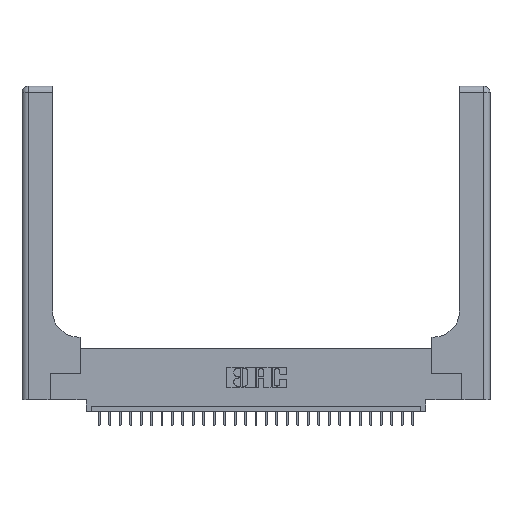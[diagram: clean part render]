
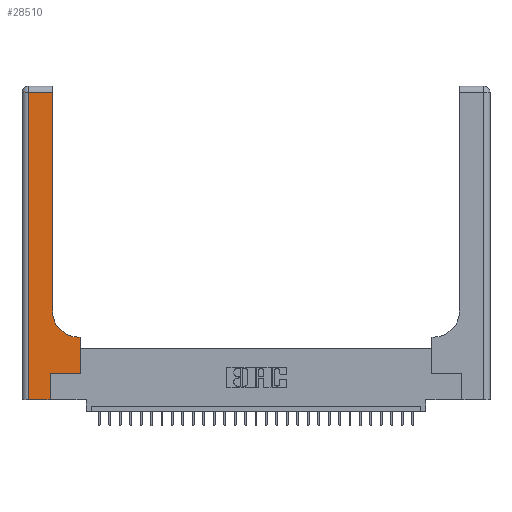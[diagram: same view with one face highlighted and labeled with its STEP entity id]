
A CAD part, top view. The second image highlights one B-rep face of the part: STEP entity #28510.
In plain terms, the highlighted planar face has unit normal (0, 0, 1).
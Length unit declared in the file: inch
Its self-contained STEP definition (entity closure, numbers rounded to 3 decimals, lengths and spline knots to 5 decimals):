
#243 = CARTESIAN_POINT ( 'NONE',  ( 0.269, 0.25, 0.37 ) ) ;
#342 = VERTEX_POINT ( 'NONE', #17810 ) ;
#638 = DIRECTION ( 'NONE',  ( 1., 0., 0. ) ) ;
#1410 = VECTOR ( 'NONE', #7088, 39.37008 ) ;
#2041 = EDGE_CURVE ( 'NONE', #10091, #8003, #2629, .T. ) ;
#2629 = LINE ( 'NONE', #28182, #18764 ) ;
#3661 = CARTESIAN_POINT ( 'NONE',  ( 0.269, 0., 0.37 ) ) ;
#4192 = ORIENTED_EDGE ( 'NONE', *, *, #15977, .T. ) ;
#4595 = EDGE_LOOP ( 'NONE', ( #4192, #26005, #29507, #8816, #28976, #13004, #23327, #13872, #29586 ) ) ;
#4893 = VECTOR ( 'NONE', #10090, 39.37008 ) ;
#5829 = DIRECTION ( 'NONE',  ( 0., -1., 0. ) ) ;
#6194 = CIRCLE ( 'NONE', #23315, 0.25 ) ;
#6256 = EDGE_CURVE ( 'NONE', #19738, #10091, #20917, .T. ) ;
#6762 = DIRECTION ( 'NONE',  ( -1., 0., 0. ) ) ;
#7088 = DIRECTION ( 'NONE',  ( -1., 0., 0. ) ) ;
#7110 = VECTOR ( 'NONE', #6762, 39.37008 ) ;
#7513 = VERTEX_POINT ( 'NONE', #15876 ) ;
#7803 = FACE_OUTER_BOUND ( 'NONE', #4595, .T. ) ;
#8003 = VERTEX_POINT ( 'NONE', #16658 ) ;
#8239 = LINE ( 'NONE', #26913, #28339 ) ;
#8816 = ORIENTED_EDGE ( 'NONE', *, *, #11697, .T. ) ;
#9368 = LINE ( 'NONE', #18712, #1410 ) ;
#9476 = CARTESIAN_POINT ( 'NONE',  ( 0.06, 2.94, 0.37 ) ) ;
#9731 = CARTESIAN_POINT ( 'NONE',  ( 0.269, 0., 0.37 ) ) ;
#10090 = DIRECTION ( 'NONE',  ( 0., 1., 0. ) ) ;
#10091 = VERTEX_POINT ( 'NONE', #243 ) ;
#10159 = CARTESIAN_POINT ( 'NONE',  ( 0.2915, 2.94, 0.37 ) ) ;
#10272 = EDGE_CURVE ( 'NONE', #14454, #7513, #6194, .T. ) ;
#11044 = LINE ( 'NONE', #30011, #7110 ) ;
#11697 = EDGE_CURVE ( 'NONE', #342, #19738, #15534, .T. ) ;
#12096 = VERTEX_POINT ( 'NONE', #9476 ) ;
#12359 = VECTOR ( 'NONE', #14035, 39.37008 ) ;
#13004 = ORIENTED_EDGE ( 'NONE', *, *, #2041, .T. ) ;
#13872 = ORIENTED_EDGE ( 'NONE', *, *, #29369, .T. ) ;
#14035 = DIRECTION ( 'NONE',  ( 0., 1., 0. ) ) ;
#14454 = VERTEX_POINT ( 'NONE', #27743 ) ;
#14844 = DIRECTION ( 'NONE',  ( 0., 0., -1. ) ) ;
#14993 = LINE ( 'NONE', #24343, #4893 ) ;
#15042 = CARTESIAN_POINT ( 'NONE',  ( 0.5415, 0.85, 0.37 ) ) ;
#15534 = LINE ( 'NONE', #25197, #23855 ) ;
#15876 = CARTESIAN_POINT ( 'NONE',  ( 0.2915, 0.85, 0.37 ) ) ;
#15977 = EDGE_CURVE ( 'NONE', #7513, #16797, #8239, .T. ) ;
#16658 = CARTESIAN_POINT ( 'NONE',  ( 0.5585, 0.25, 0.37 ) ) ;
#16797 = VERTEX_POINT ( 'NONE', #10159 ) ;
#17145 = PLANE ( 'NONE',  #23704 ) ;
#17810 = CARTESIAN_POINT ( 'NONE',  ( 0.06, 0., 0.37 ) ) ;
#18712 = CARTESIAN_POINT ( 'NONE',  ( 0., 2.94, 0.37 ) ) ;
#18764 = VECTOR ( 'NONE', #638, 39.37008 ) ;
#19738 = VERTEX_POINT ( 'NONE', #3661 ) ;
#20246 = EDGE_CURVE ( 'NONE', #16797, #12096, #9368, .T. ) ;
#20912 = CARTESIAN_POINT ( 'NONE',  ( 0.5585, 0.6, 0.37 ) ) ;
#20917 = LINE ( 'NONE', #9731, #12359 ) ;
#21901 = CARTESIAN_POINT ( 'NONE',  ( 0.06, 3., 0.37 ) ) ;
#21943 = EDGE_CURVE ( 'NONE', #8003, #23517, #14993, .T. ) ;
#23247 = VECTOR ( 'NONE', #5829, 39.37008 ) ;
#23315 = AXIS2_PLACEMENT_3D ( 'NONE', #15042, #28970, #28377 ) ;
#23327 = ORIENTED_EDGE ( 'NONE', *, *, #21943, .T. ) ;
#23517 = VERTEX_POINT ( 'NONE', #20912 ) ;
#23704 = AXIS2_PLACEMENT_3D ( 'NONE', #26479, #14844, #24202 ) ;
#23855 = VECTOR ( 'NONE', #27774, 39.37008 ) ;
#24202 = DIRECTION ( 'NONE',  ( -1., 0., 0. ) ) ;
#24343 = CARTESIAN_POINT ( 'NONE',  ( 0.5585, 0.25, 0.37 ) ) ;
#25197 = CARTESIAN_POINT ( 'NONE',  ( 0., 0., 0.37 ) ) ;
#26005 = ORIENTED_EDGE ( 'NONE', *, *, #20246, .T. ) ;
#26479 = CARTESIAN_POINT ( 'NONE',  ( 0., 3., 0.37 ) ) ;
#26637 = LINE ( 'NONE', #21901, #23247 ) ;
#26767 = DIRECTION ( 'NONE',  ( 0., 1., 0. ) ) ;
#26913 = CARTESIAN_POINT ( 'NONE',  ( 0.2915, 3., 0.37 ) ) ;
#27743 = CARTESIAN_POINT ( 'NONE',  ( 0.5415, 0.6, 0.37 ) ) ;
#27774 = DIRECTION ( 'NONE',  ( 1., 0., 0. ) ) ;
#28182 = CARTESIAN_POINT ( 'NONE',  ( 0.269, 0.25, 0.37 ) ) ;
#28339 = VECTOR ( 'NONE', #26767, 39.37008 ) ;
#28377 = DIRECTION ( 'NONE',  ( 1., 0., 0. ) ) ;
#28510 = ADVANCED_FACE ( 'NONE', ( #7803 ), #17145, .F. ) ;
#28970 = DIRECTION ( 'NONE',  ( 0., 0., -1. ) ) ;
#28976 = ORIENTED_EDGE ( 'NONE', *, *, #6256, .T. ) ;
#29369 = EDGE_CURVE ( 'NONE', #23517, #14454, #11044, .T. ) ;
#29507 = ORIENTED_EDGE ( 'NONE', *, *, #29564, .T. ) ;
#29564 = EDGE_CURVE ( 'NONE', #12096, #342, #26637, .T. ) ;
#29586 = ORIENTED_EDGE ( 'NONE', *, *, #10272, .T. ) ;
#30011 = CARTESIAN_POINT ( 'NONE',  ( 0.2915, 0.6, 0.37 ) ) ;
